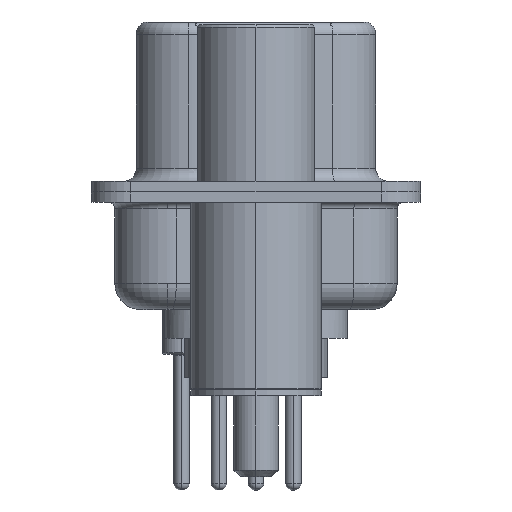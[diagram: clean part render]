
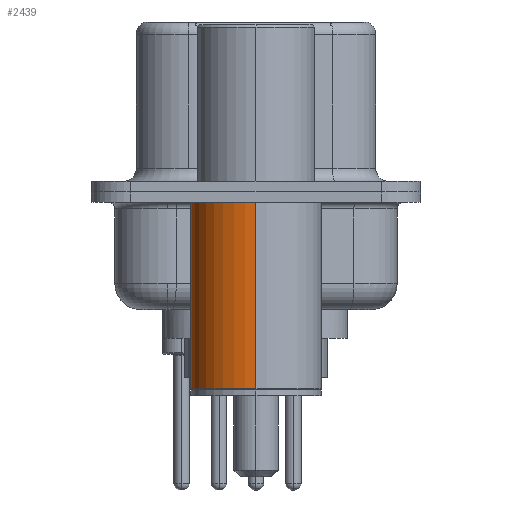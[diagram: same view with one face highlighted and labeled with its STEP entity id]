
A CAD part, left-side view. The second image highlights one B-rep face of the part: STEP entity #2439.
In plain terms, the highlighted cylindrical face has radius 2.5 mm (diameter 5 mm), a partial arc.
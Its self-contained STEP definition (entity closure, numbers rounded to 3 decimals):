
#281 = ORIENTED_EDGE ( 'NONE', *, *, #21947, .T. ) ;
#491 = CARTESIAN_POINT ( 'NONE',  ( 2.5, 0., -7.525 ) ) ;
#1321 = CARTESIAN_POINT ( 'NONE',  ( -2.5, 0., -7.525 ) ) ;
#2107 = DIRECTION ( 'NONE',  ( 1., 0., 0. ) ) ;
#2439 = ADVANCED_FACE ( 'NONE', ( #8716 ), #3087, .T. ) ;
#2877 = EDGE_CURVE ( 'NONE', #17869, #22834, #16953, .T. ) ;
#3042 = VERTEX_POINT ( 'NONE', #491 ) ;
#3087 = CYLINDRICAL_SURFACE ( 'NONE', #20761, 2.5 ) ;
#3286 = CARTESIAN_POINT ( 'NONE',  ( 2.5, 0., 0.581 ) ) ;
#3298 = CARTESIAN_POINT ( 'NONE',  ( -2.5, 0., 0.581 ) ) ;
#3524 = ORIENTED_EDGE ( 'NONE', *, *, #5506, .F. ) ;
#4079 = LINE ( 'NONE', #3298, #14636 ) ;
#4155 = ORIENTED_EDGE ( 'NONE', *, *, #2877, .F. ) ;
#5421 = DIRECTION ( 'NONE',  ( 0., 0., 1. ) ) ;
#5506 = EDGE_CURVE ( 'NONE', #3042, #17869, #16835, .T. ) ;
#5566 = VECTOR ( 'NONE', #14821, 1000. ) ;
#7199 = CARTESIAN_POINT ( 'NONE',  ( 2.5, 0., -0.4 ) ) ;
#8716 = FACE_OUTER_BOUND ( 'NONE', #19495, .T. ) ;
#9790 = AXIS2_PLACEMENT_3D ( 'NONE', #11609, #26148, #10139 ) ;
#10139 = DIRECTION ( 'NONE',  ( 1., 0., 0. ) ) ;
#11609 = CARTESIAN_POINT ( 'NONE',  ( 0., 0., -0.4 ) ) ;
#11664 = EDGE_CURVE ( 'NONE', #3042, #13420, #25166, .T. ) ;
#12158 = CARTESIAN_POINT ( 'NONE',  ( -2.5, 0., -0.4 ) ) ;
#13420 = VERTEX_POINT ( 'NONE', #1321 ) ;
#14636 = VECTOR ( 'NONE', #5421, 1000. ) ;
#14727 = DIRECTION ( 'NONE',  ( 0., 0., 1. ) ) ;
#14821 = DIRECTION ( 'NONE',  ( 0., 0., 1. ) ) ;
#15648 = CARTESIAN_POINT ( 'NONE',  ( 0., 0., 0.581 ) ) ;
#16315 = AXIS2_PLACEMENT_3D ( 'NONE', #27453, #14727, #2107 ) ;
#16835 = LINE ( 'NONE', #3286, #5566 ) ;
#16953 = CIRCLE ( 'NONE', #9790, 2.5 ) ;
#17869 = VERTEX_POINT ( 'NONE', #7199 ) ;
#18224 = ORIENTED_EDGE ( 'NONE', *, *, #11664, .T. ) ;
#19495 = EDGE_LOOP ( 'NONE', ( #18224, #281, #4155, #3524 ) ) ;
#20159 = DIRECTION ( 'NONE',  ( 0., 0., 1. ) ) ;
#20761 = AXIS2_PLACEMENT_3D ( 'NONE', #15648, #20159, #22181 ) ;
#21947 = EDGE_CURVE ( 'NONE', #13420, #22834, #4079, .T. ) ;
#22181 = DIRECTION ( 'NONE',  ( 1., 0., 0. ) ) ;
#22834 = VERTEX_POINT ( 'NONE', #12158 ) ;
#25166 = CIRCLE ( 'NONE', #16315, 2.5 ) ;
#26148 = DIRECTION ( 'NONE',  ( 0., 0., 1. ) ) ;
#27453 = CARTESIAN_POINT ( 'NONE',  ( 0., 0., -7.525 ) ) ;
